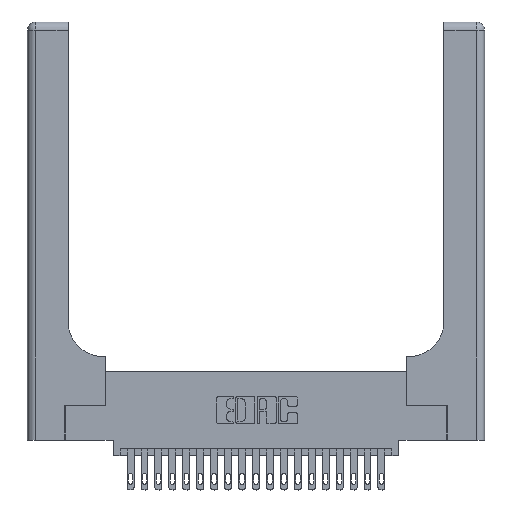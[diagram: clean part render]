
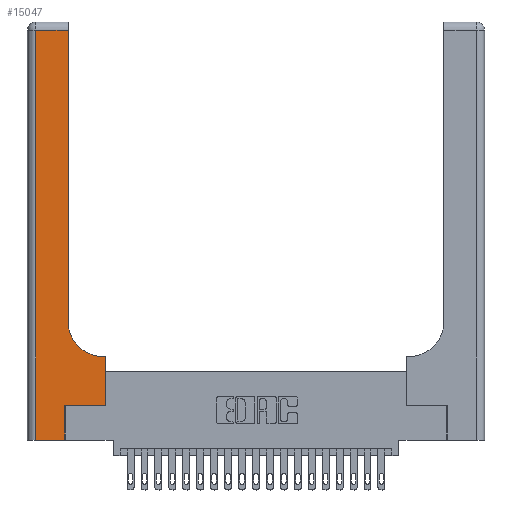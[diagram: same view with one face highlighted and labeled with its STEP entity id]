
A CAD part, top view. The second image highlights one B-rep face of the part: STEP entity #15047.
In plain terms, the highlighted planar face has unit normal (0, 0, 1).
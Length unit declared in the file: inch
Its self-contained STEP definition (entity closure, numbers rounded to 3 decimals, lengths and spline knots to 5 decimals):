
#500 = DIRECTION ( 'NONE',  ( -1., 0., 0. ) ) ;
#913 = DIRECTION ( 'NONE',  ( 0., 1., 0. ) ) ;
#1690 = DIRECTION ( 'NONE',  ( 0., 1., 0. ) ) ;
#2050 = DIRECTION ( 'NONE',  ( 0., 0., -1. ) ) ;
#2451 = FACE_OUTER_BOUND ( 'NONE', #12630, .T. ) ;
#2513 = EDGE_CURVE ( 'NONE', #6463, #18833, #9497, .T. ) ;
#2846 = LINE ( 'NONE', #22874, #7874 ) ;
#2861 = VECTOR ( 'NONE', #500, 39.37008 ) ;
#2989 = VECTOR ( 'NONE', #19258, 39.37008 ) ;
#3275 = AXIS2_PLACEMENT_3D ( 'NONE', #8553, #22926, #8054 ) ;
#3443 = LINE ( 'NONE', #13349, #15508 ) ;
#4125 = AXIS2_PLACEMENT_3D ( 'NONE', #12763, #2050, #14423 ) ;
#4496 = DIRECTION ( 'NONE',  ( 0., -1., 0. ) ) ;
#5548 = EDGE_CURVE ( 'NONE', #20665, #16893, #7711, .T. ) ;
#5737 = ORIENTED_EDGE ( 'NONE', *, *, #22003, .T. ) ;
#6032 = CARTESIAN_POINT ( 'NONE',  ( 0.5585, 0.6, 0.37 ) ) ;
#6355 = CARTESIAN_POINT ( 'NONE',  ( 0.2915, 2.94, 0.37 ) ) ;
#6463 = VERTEX_POINT ( 'NONE', #13045 ) ;
#6958 = VECTOR ( 'NONE', #4496, 39.37008 ) ;
#7234 = ORIENTED_EDGE ( 'NONE', *, *, #9198, .T. ) ;
#7268 = ORIENTED_EDGE ( 'NONE', *, *, #5548, .T. ) ;
#7604 = VERTEX_POINT ( 'NONE', #6032 ) ;
#7711 = LINE ( 'NONE', #11414, #2989 ) ;
#7792 = VERTEX_POINT ( 'NONE', #12484 ) ;
#7874 = VECTOR ( 'NONE', #1690, 39.37008 ) ;
#8000 = LINE ( 'NONE', #9201, #12511 ) ;
#8054 = DIRECTION ( 'NONE',  ( -1., 0., 0. ) ) ;
#8146 = VERTEX_POINT ( 'NONE', #14785 ) ;
#8315 = CARTESIAN_POINT ( 'NONE',  ( 0.06, 3., 0.37 ) ) ;
#8464 = CARTESIAN_POINT ( 'NONE',  ( 0.5585, 0.25, 0.37 ) ) ;
#8470 = VECTOR ( 'NONE', #10985, 39.37008 ) ;
#8553 = CARTESIAN_POINT ( 'NONE',  ( 0., 3., 0.37 ) ) ;
#9198 = EDGE_CURVE ( 'NONE', #9814, #7792, #20738, .T. ) ;
#9201 = CARTESIAN_POINT ( 'NONE',  ( 0., 2.94, 0.37 ) ) ;
#9497 = CIRCLE ( 'NONE', #4125, 0.25 ) ;
#9814 = VERTEX_POINT ( 'NONE', #13830 ) ;
#10985 = DIRECTION ( 'NONE',  ( 0., 1., 0. ) ) ;
#11414 = CARTESIAN_POINT ( 'NONE',  ( 0.269, 0.25, 0.37 ) ) ;
#11564 = CARTESIAN_POINT ( 'NONE',  ( 0.2915, 0.85, 0.37 ) ) ;
#11896 = DIRECTION ( 'NONE',  ( -1., 0., 0. ) ) ;
#11936 = EDGE_CURVE ( 'NONE', #8146, #20665, #13832, .T. ) ;
#12280 = ORIENTED_EDGE ( 'NONE', *, *, #11936, .T. ) ;
#12484 = CARTESIAN_POINT ( 'NONE',  ( 0.06, 0., 0.37 ) ) ;
#12511 = VECTOR ( 'NONE', #11896, 39.37008 ) ;
#12630 = EDGE_LOOP ( 'NONE', ( #5737, #22780, #7234, #23138, #12280, #7268, #19066, #15176, #23047 ) ) ;
#12763 = CARTESIAN_POINT ( 'NONE',  ( 0.5415, 0.85, 0.37 ) ) ;
#12861 = EDGE_CURVE ( 'NONE', #16893, #7604, #2846, .T. ) ;
#13045 = CARTESIAN_POINT ( 'NONE',  ( 0.5415, 0.6, 0.37 ) ) ;
#13349 = CARTESIAN_POINT ( 'NONE',  ( 0., 0., 0.37 ) ) ;
#13830 = CARTESIAN_POINT ( 'NONE',  ( 0.06, 2.94, 0.37 ) ) ;
#13832 = LINE ( 'NONE', #22427, #20319 ) ;
#14423 = DIRECTION ( 'NONE',  ( 1., 0., 0. ) ) ;
#14785 = CARTESIAN_POINT ( 'NONE',  ( 0.269, 0., 0.37 ) ) ;
#15047 = ADVANCED_FACE ( 'NONE', ( #2451 ), #20647, .F. ) ;
#15176 = ORIENTED_EDGE ( 'NONE', *, *, #23111, .T. ) ;
#15483 = LINE ( 'NONE', #18287, #2861 ) ;
#15508 = VECTOR ( 'NONE', #20958, 39.37008 ) ;
#16053 = LINE ( 'NONE', #16547, #8470 ) ;
#16106 = EDGE_CURVE ( 'NONE', #19776, #9814, #8000, .T. ) ;
#16547 = CARTESIAN_POINT ( 'NONE',  ( 0.2915, 3., 0.37 ) ) ;
#16893 = VERTEX_POINT ( 'NONE', #8464 ) ;
#18287 = CARTESIAN_POINT ( 'NONE',  ( 0.2915, 0.6, 0.37 ) ) ;
#18833 = VERTEX_POINT ( 'NONE', #11564 ) ;
#19066 = ORIENTED_EDGE ( 'NONE', *, *, #12861, .T. ) ;
#19258 = DIRECTION ( 'NONE',  ( 1., 0., 0. ) ) ;
#19776 = VERTEX_POINT ( 'NONE', #6355 ) ;
#20319 = VECTOR ( 'NONE', #913, 39.37008 ) ;
#20647 = PLANE ( 'NONE',  #3275 ) ;
#20665 = VERTEX_POINT ( 'NONE', #21249 ) ;
#20738 = LINE ( 'NONE', #8315, #6958 ) ;
#20958 = DIRECTION ( 'NONE',  ( 1., 0., 0. ) ) ;
#21249 = CARTESIAN_POINT ( 'NONE',  ( 0.269, 0.25, 0.37 ) ) ;
#22003 = EDGE_CURVE ( 'NONE', #18833, #19776, #16053, .T. ) ;
#22427 = CARTESIAN_POINT ( 'NONE',  ( 0.269, 0., 0.37 ) ) ;
#22700 = EDGE_CURVE ( 'NONE', #7792, #8146, #3443, .T. ) ;
#22780 = ORIENTED_EDGE ( 'NONE', *, *, #16106, .T. ) ;
#22874 = CARTESIAN_POINT ( 'NONE',  ( 0.5585, 0.25, 0.37 ) ) ;
#22926 = DIRECTION ( 'NONE',  ( 0., 0., -1. ) ) ;
#23047 = ORIENTED_EDGE ( 'NONE', *, *, #2513, .T. ) ;
#23111 = EDGE_CURVE ( 'NONE', #7604, #6463, #15483, .T. ) ;
#23138 = ORIENTED_EDGE ( 'NONE', *, *, #22700, .T. ) ;
